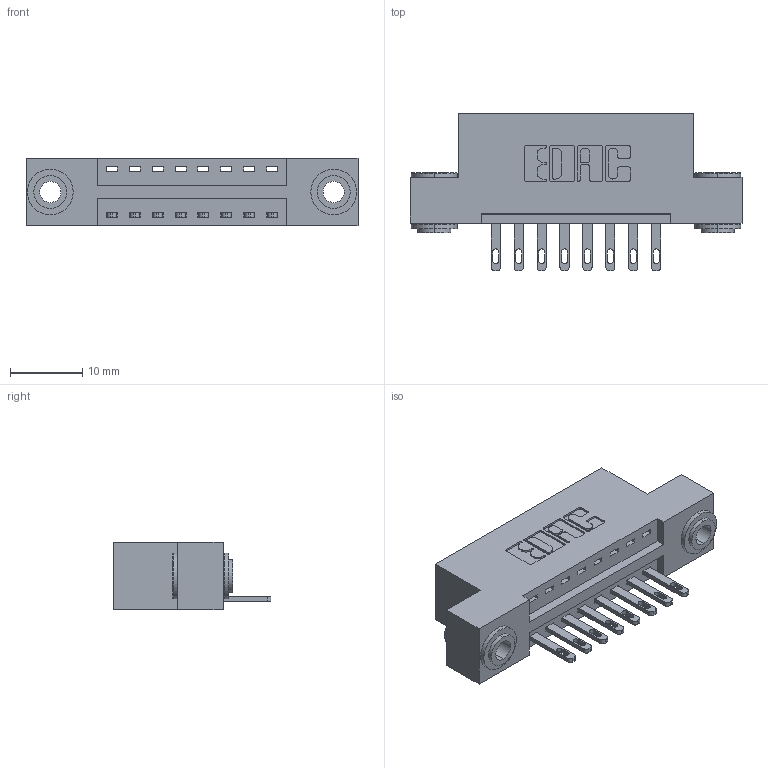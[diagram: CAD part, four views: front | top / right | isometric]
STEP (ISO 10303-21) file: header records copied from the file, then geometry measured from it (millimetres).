
FILE_DESCRIPTION (( 'STEP AP203' ), '1' );
FILE_NAME ('346-008-500-103.STEP', '2022-05-04T20:33:03', ( '' ), ( '' ), 'SwSTEP 2.0', 'SolidWorks 2020', '' );
FILE_SCHEMA (( 'CONFIG_CONTROL_DESIGN' ));
Length unit declared in the file: inch
Products named in the file (4): 346 Part_Flush Mounting Lugs - 0.156 Dia-TH; 345-292-001_345-293-100; 345-250-002_345-250-002-102; 346-008-500-103
Assembly tree (11 placements, depth 2):
  346-008-500-103
    346 Part_Flush Mounting Lugs - 0.156 Dia-TH
    345-292-001_345-293-100  x8
    345-250-002_345-250-002-102  x2
Bounding box: 45.97 x 21.84 x 9.4 mm (x, y, z)
Volume: 4172.7 mm3; surface area: 5118.6 mm2
Topology: 11 solids, 11 shells, 606 faces, 1785 edges, 1186 vertices
Faces by surface type: plane 372, cylinder 226, cone 8
Entity records: 10538 total; most frequent: CARTESIAN_POINT 1797, ORIENTED_EDGE 1730, DIRECTION 1659, EDGE_CURVE 865, VECTOR 673, LINE 673, VERTEX_POINT 574, AXIS2_PLACEMENT_3D 493
